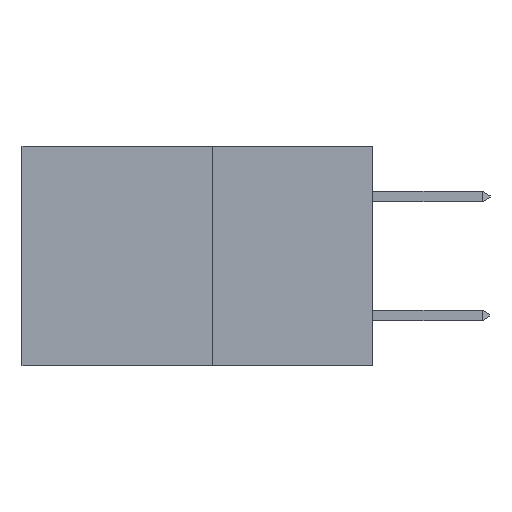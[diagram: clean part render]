
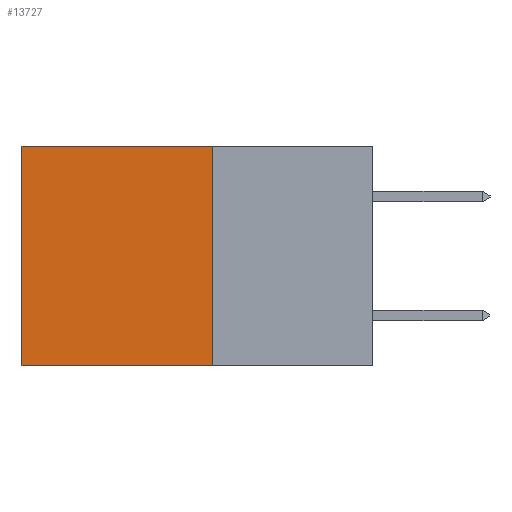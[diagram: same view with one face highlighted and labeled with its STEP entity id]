
A CAD part, left-side view. The second image highlights one B-rep face of the part: STEP entity #13727.
In plain terms, the highlighted planar face has unit normal (-1, 0, 0).
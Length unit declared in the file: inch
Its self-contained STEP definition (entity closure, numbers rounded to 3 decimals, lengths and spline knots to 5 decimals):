
#190 = LINE ( 'NONE', #2286, #6986 ) ;
#265 = VERTEX_POINT ( 'NONE', #326 ) ;
#326 = CARTESIAN_POINT ( 'NONE',  ( 0.277, 0.59, 0. ) ) ;
#2110 = VECTOR ( 'NONE', #6601, 39.37008 ) ;
#2286 = CARTESIAN_POINT ( 'NONE',  ( 0.277, 0.27, -0.37 ) ) ;
#2767 = PLANE ( 'NONE',  #13980 ) ;
#2994 = ORIENTED_EDGE ( 'NONE', *, *, #14517, .T. ) ;
#3716 = EDGE_LOOP ( 'NONE', ( #15195, #5793, #10574, #2994 ) ) ;
#4254 = DIRECTION ( 'NONE',  ( 1., 0., 0. ) ) ;
#4932 = LINE ( 'NONE', #8963, #2110 ) ;
#5186 = VECTOR ( 'NONE', #13873, 39.37008 ) ;
#5793 = ORIENTED_EDGE ( 'NONE', *, *, #13424, .F. ) ;
#5836 = EDGE_CURVE ( 'NONE', #13260, #11810, #4932, .T. ) ;
#5844 = VECTOR ( 'NONE', #8780, 39.37008 ) ;
#6403 = EDGE_CURVE ( 'NONE', #265, #13617, #15230, .T. ) ;
#6601 = DIRECTION ( 'NONE',  ( 0., 0., -1. ) ) ;
#6986 = VECTOR ( 'NONE', #9456, 39.37008 ) ;
#7597 = CARTESIAN_POINT ( 'NONE',  ( 0.277, 0.59, -0.37 ) ) ;
#8363 = LINE ( 'NONE', #12702, #5186 ) ;
#8780 = DIRECTION ( 'NONE',  ( 0., 0., -1. ) ) ;
#8963 = CARTESIAN_POINT ( 'NONE',  ( 0.277, 0.27, -0.37 ) ) ;
#9456 = DIRECTION ( 'NONE',  ( 0., 1., 0. ) ) ;
#10574 = ORIENTED_EDGE ( 'NONE', *, *, #5836, .F. ) ;
#10998 = CARTESIAN_POINT ( 'NONE',  ( 0.277, 0.59, -0.37 ) ) ;
#11243 = FACE_OUTER_BOUND ( 'NONE', #3716, .T. ) ;
#11354 = CARTESIAN_POINT ( 'NONE',  ( 0.277, 0.27, -0.37 ) ) ;
#11367 = CARTESIAN_POINT ( 'NONE',  ( 0.277, 0.27, 0. ) ) ;
#11810 = VERTEX_POINT ( 'NONE', #15202 ) ;
#12520 = DIRECTION ( 'NONE',  ( 0., 0., -1. ) ) ;
#12702 = CARTESIAN_POINT ( 'NONE',  ( 0.277, 0.27, 0. ) ) ;
#13260 = VERTEX_POINT ( 'NONE', #11367 ) ;
#13424 = EDGE_CURVE ( 'NONE', #11810, #13617, #190, .T. ) ;
#13617 = VERTEX_POINT ( 'NONE', #10998 ) ;
#13727 = ADVANCED_FACE ( 'NONE', ( #11243 ), #2767, .F. ) ;
#13873 = DIRECTION ( 'NONE',  ( 0., 1., 0. ) ) ;
#13980 = AXIS2_PLACEMENT_3D ( 'NONE', #11354, #4254, #12520 ) ;
#14517 = EDGE_CURVE ( 'NONE', #13260, #265, #8363, .T. ) ;
#15195 = ORIENTED_EDGE ( 'NONE', *, *, #6403, .T. ) ;
#15202 = CARTESIAN_POINT ( 'NONE',  ( 0.277, 0.27, -0.37 ) ) ;
#15230 = LINE ( 'NONE', #7597, #5844 ) ;
